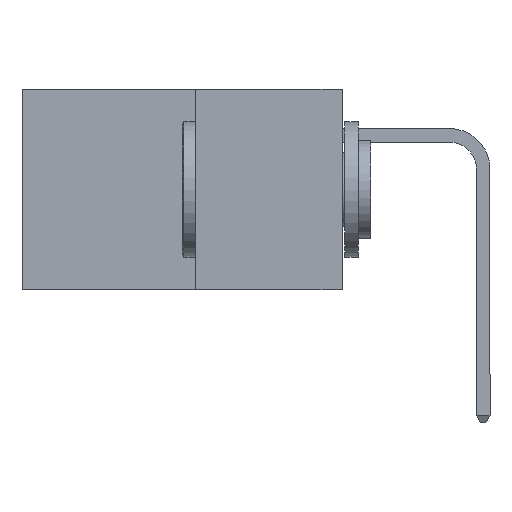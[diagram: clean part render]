
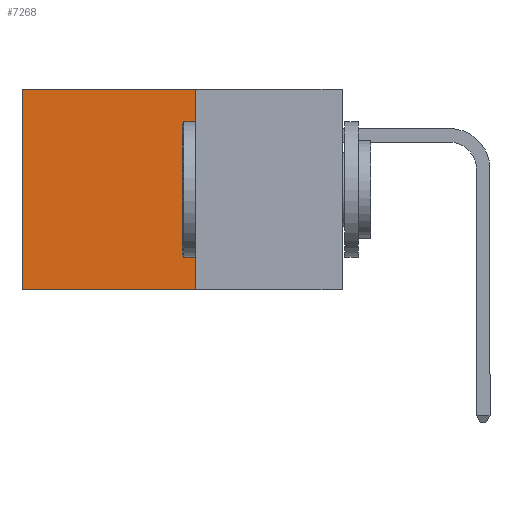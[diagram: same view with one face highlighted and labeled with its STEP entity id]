
A CAD part, left-side view. The second image highlights one B-rep face of the part: STEP entity #7268.
In plain terms, the highlighted planar face has unit normal (-1, 0, 0).
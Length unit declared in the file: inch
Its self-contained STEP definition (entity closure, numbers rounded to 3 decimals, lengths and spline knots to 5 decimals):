
#557 = CARTESIAN_POINT ( 'NONE',  ( 0.277, 0.27, 0. ) ) ;
#700 = LINE ( 'NONE', #8817, #6305 ) ;
#837 = EDGE_LOOP ( 'NONE', ( #5132, #6076, #6994, #4522 ) ) ;
#1018 = VECTOR ( 'NONE', #4406, 39.37008 ) ;
#1359 = CARTESIAN_POINT ( 'NONE',  ( 0.277, 0.27, -0.37 ) ) ;
#1375 = DIRECTION ( 'NONE',  ( 0., 0., -1. ) ) ;
#1450 = DIRECTION ( 'NONE',  ( 0., 0., -1. ) ) ;
#1459 = DIRECTION ( 'NONE',  ( 1., 0., 0. ) ) ;
#1535 = LINE ( 'NONE', #6815, #3786 ) ;
#1560 = CARTESIAN_POINT ( 'NONE',  ( 0.277, 0.27, -0.37 ) ) ;
#1622 = PLANE ( 'NONE',  #7572 ) ;
#2030 = CARTESIAN_POINT ( 'NONE',  ( 0.277, 0.27, 0. ) ) ;
#2348 = VERTEX_POINT ( 'NONE', #8258 ) ;
#2521 = EDGE_CURVE ( 'NONE', #5141, #6409, #700, .T. ) ;
#2615 = EDGE_CURVE ( 'NONE', #2348, #6409, #1535, .T. ) ;
#2849 = VERTEX_POINT ( 'NONE', #2030 ) ;
#3162 = VECTOR ( 'NONE', #1375, 39.37008 ) ;
#3231 = FACE_OUTER_BOUND ( 'NONE', #837, .T. ) ;
#3786 = VECTOR ( 'NONE', #5397, 39.37008 ) ;
#4116 = EDGE_CURVE ( 'NONE', #2849, #2348, #5468, .T. ) ;
#4406 = DIRECTION ( 'NONE',  ( 0., 1., 0. ) ) ;
#4522 = ORIENTED_EDGE ( 'NONE', *, *, #8345, .T. ) ;
#5132 = ORIENTED_EDGE ( 'NONE', *, *, #2521, .T. ) ;
#5141 = VERTEX_POINT ( 'NONE', #7806 ) ;
#5397 = DIRECTION ( 'NONE',  ( 0., 1., 0. ) ) ;
#5468 = LINE ( 'NONE', #1359, #3162 ) ;
#5951 = CARTESIAN_POINT ( 'NONE',  ( 0.277, 0.59, -0.37 ) ) ;
#6076 = ORIENTED_EDGE ( 'NONE', *, *, #2615, .F. ) ;
#6305 = VECTOR ( 'NONE', #9217, 39.37008 ) ;
#6409 = VERTEX_POINT ( 'NONE', #5951 ) ;
#6815 = CARTESIAN_POINT ( 'NONE',  ( 0.277, 0.27, -0.37 ) ) ;
#6994 = ORIENTED_EDGE ( 'NONE', *, *, #4116, .F. ) ;
#7268 = ADVANCED_FACE ( 'NONE', ( #3231 ), #1622, .F. ) ;
#7572 = AXIS2_PLACEMENT_3D ( 'NONE', #1560, #1459, #1450 ) ;
#7806 = CARTESIAN_POINT ( 'NONE',  ( 0.277, 0.59, 0. ) ) ;
#8258 = CARTESIAN_POINT ( 'NONE',  ( 0.277, 0.27, -0.37 ) ) ;
#8345 = EDGE_CURVE ( 'NONE', #2849, #5141, #9195, .T. ) ;
#8817 = CARTESIAN_POINT ( 'NONE',  ( 0.277, 0.59, -0.37 ) ) ;
#9195 = LINE ( 'NONE', #557, #1018 ) ;
#9217 = DIRECTION ( 'NONE',  ( 0., 0., -1. ) ) ;
